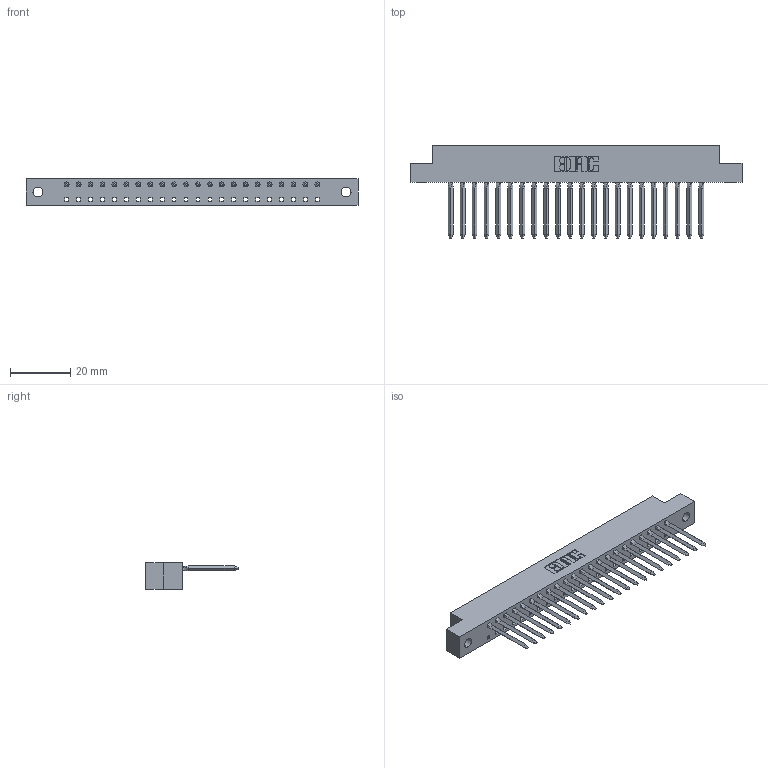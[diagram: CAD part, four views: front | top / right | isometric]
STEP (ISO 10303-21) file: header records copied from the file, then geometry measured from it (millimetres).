
FILE_DESCRIPTION (( 'STEP AP203' ), '1' );
FILE_NAME ('338-022-541-102.STEP', '2020-03-24T17:44:16', ( '' ), ( '' ), 'SwSTEP 2.0', 'SolidWorks 2016', '' );
FILE_SCHEMA (( 'CONFIG_CONTROL_DESIGN' ));
Length unit declared in the file: inch
Products named in the file (3): 338-290-001_541; 338-210-001_338-210-022-002; 338-022-541-102
Assembly tree (23 placements, depth 2):
  338-022-541-102
    338-210-001_338-210-022-002
    338-290-001_541  x22
Bounding box: 110.19 x 30.56 x 8.71 mm (x, y, z)
Volume: 7675.8 mm3; surface area: 12101.8 mm2
Topology: 23 solids, 23 shells, 2140 faces, 5905 edges, 3774 vertices
Faces by surface type: plane 1480, cylinder 572, bspline 88
Entity records: 44278 total; most frequent: CARTESIAN_POINT 8922, ORIENTED_EDGE 7484, DIRECTION 6973, EDGE_CURVE 3742, VECTOR 2779, LINE 2779, VERTEX_POINT 2430, AXIS2_PLACEMENT_3D 2097
